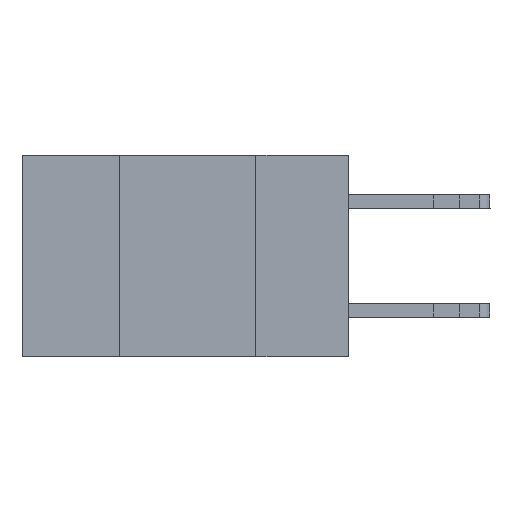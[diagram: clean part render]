
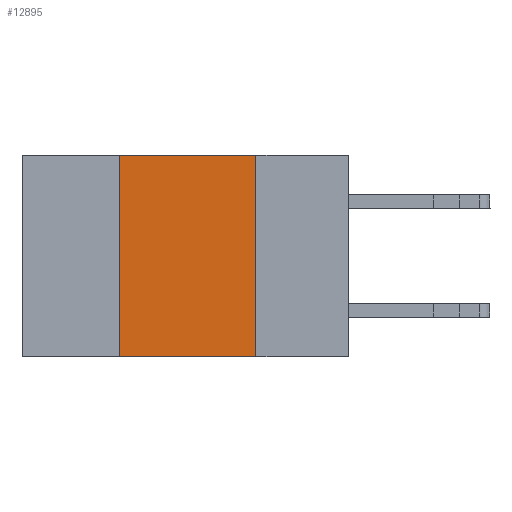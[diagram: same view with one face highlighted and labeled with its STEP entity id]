
A CAD part, left-side view. The second image highlights one B-rep face of the part: STEP entity #12895.
In plain terms, the highlighted planar face has unit normal (-1, 0, 0).
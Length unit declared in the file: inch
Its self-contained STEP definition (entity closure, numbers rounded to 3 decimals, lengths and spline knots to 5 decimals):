
#548 = DIRECTION ( 'NONE',  ( 0., 0., 1. ) ) ;
#1214 = LINE ( 'NONE', #8480, #8510 ) ;
#1233 = VERTEX_POINT ( 'NONE', #8905 ) ;
#1362 = VERTEX_POINT ( 'NONE', #15851 ) ;
#1508 = DIRECTION ( 'NONE',  ( 1., 0., 0. ) ) ;
#1746 = EDGE_CURVE ( 'NONE', #1233, #1362, #15339, .T. ) ;
#2318 = VECTOR ( 'NONE', #10881, 39.37008 ) ;
#2819 = ORIENTED_EDGE ( 'NONE', *, *, #1746, .F. ) ;
#2892 = CARTESIAN_POINT ( 'NONE',  ( 0., 0.17, 0. ) ) ;
#3173 = VECTOR ( 'NONE', #548, 39.37008 ) ;
#4673 = CARTESIAN_POINT ( 'NONE',  ( 0., 0.6, -0.37 ) ) ;
#4927 = EDGE_LOOP ( 'NONE', ( #5766, #14046, #2819, #15079 ) ) ;
#5766 = ORIENTED_EDGE ( 'NONE', *, *, #13684, .F. ) ;
#5786 = LINE ( 'NONE', #4673, #2318 ) ;
#6201 = DIRECTION ( 'NONE',  ( 0., 0., -1. ) ) ;
#7416 = PLANE ( 'NONE',  #9307 ) ;
#8480 = CARTESIAN_POINT ( 'NONE',  ( 0., 0.17, -0.37 ) ) ;
#8510 = VECTOR ( 'NONE', #15845, 39.37008 ) ;
#8905 = CARTESIAN_POINT ( 'NONE',  ( 0., 0.42, -0.37 ) ) ;
#9307 = AXIS2_PLACEMENT_3D ( 'NONE', #13721, #1508, #6201 ) ;
#10335 = CARTESIAN_POINT ( 'NONE',  ( 0., 0.17, -0.37 ) ) ;
#10881 = DIRECTION ( 'NONE',  ( 0., -1., 0. ) ) ;
#10960 = EDGE_CURVE ( 'NONE', #1233, #13295, #5786, .T. ) ;
#11699 = CARTESIAN_POINT ( 'NONE',  ( 0., 0.42, -0.37 ) ) ;
#12427 = VECTOR ( 'NONE', #15495, 39.37008 ) ;
#12661 = VERTEX_POINT ( 'NONE', #2892 ) ;
#12708 = EDGE_CURVE ( 'NONE', #1362, #12661, #13974, .T. ) ;
#12895 = ADVANCED_FACE ( 'NONE', ( #14932 ), #7416, .F. ) ;
#13063 = CARTESIAN_POINT ( 'NONE',  ( 0., 0.6, 0. ) ) ;
#13295 = VERTEX_POINT ( 'NONE', #10335 ) ;
#13684 = EDGE_CURVE ( 'NONE', #12661, #13295, #1214, .T. ) ;
#13721 = CARTESIAN_POINT ( 'NONE',  ( 0., 0.6, 0. ) ) ;
#13974 = LINE ( 'NONE', #13063, #12427 ) ;
#14046 = ORIENTED_EDGE ( 'NONE', *, *, #12708, .F. ) ;
#14932 = FACE_OUTER_BOUND ( 'NONE', #4927, .T. ) ;
#15079 = ORIENTED_EDGE ( 'NONE', *, *, #10960, .T. ) ;
#15339 = LINE ( 'NONE', #11699, #3173 ) ;
#15495 = DIRECTION ( 'NONE',  ( 0., -1., 0. ) ) ;
#15845 = DIRECTION ( 'NONE',  ( 0., 0., -1. ) ) ;
#15851 = CARTESIAN_POINT ( 'NONE',  ( 0., 0.42, 0. ) ) ;
